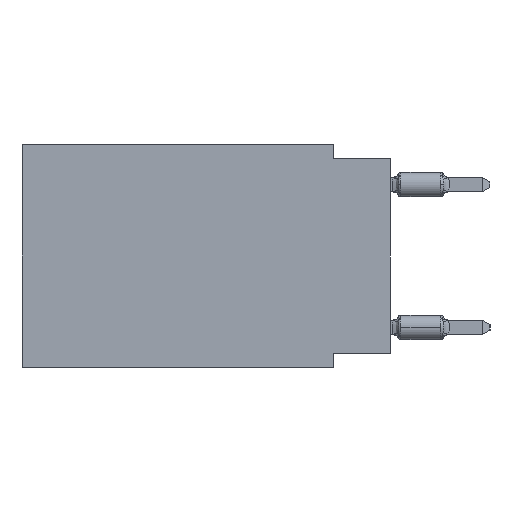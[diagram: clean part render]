
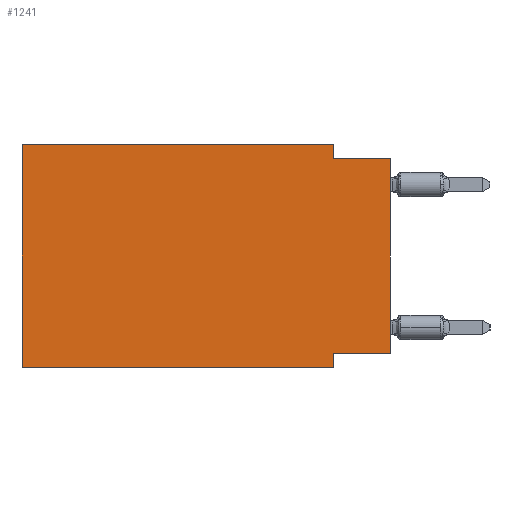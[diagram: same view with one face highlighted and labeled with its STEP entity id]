
A CAD part, left-side view. The second image highlights one B-rep face of the part: STEP entity #1241.
In plain terms, the highlighted planar face has unit normal (-1, 0, 0).
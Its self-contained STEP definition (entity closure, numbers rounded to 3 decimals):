
#1184 = DIRECTION ( 'NONE',  ( 0., 0., -1. ) ) ;
#1241 = ADVANCED_FACE ( 'NONE', ( #9945 ), #9842, .F. ) ;
#1271 = VERTEX_POINT ( 'NONE', #1636 ) ;
#1636 = CARTESIAN_POINT ( 'NONE',  ( 0., 16.383, -9.906 ) ) ;
#2718 = ORIENTED_EDGE ( 'NONE', *, *, #7008, .F. ) ;
#3216 = DIRECTION ( 'NONE',  ( 0., -1., 0. ) ) ;
#3234 = LINE ( 'NONE', #7346, #17052 ) ;
#3981 = ORIENTED_EDGE ( 'NONE', *, *, #22435, .F. ) ;
#5468 = CARTESIAN_POINT ( 'NONE',  ( 0., 2.54, -9.906 ) ) ;
#5648 = EDGE_CURVE ( 'NONE', #15885, #8867, #14203, .T. ) ;
#6075 = ORIENTED_EDGE ( 'NONE', *, *, #6110, .F. ) ;
#6110 = EDGE_CURVE ( 'NONE', #1271, #9626, #15998, .T. ) ;
#6120 = VERTEX_POINT ( 'NONE', #14290 ) ;
#6160 = VECTOR ( 'NONE', #12647, 1000. ) ;
#6846 = VECTOR ( 'NONE', #15282, 1000. ) ;
#6940 = DIRECTION ( 'NONE',  ( 0., -1., 0. ) ) ;
#7008 = EDGE_CURVE ( 'NONE', #9626, #15885, #8677, .T. ) ;
#7224 = DIRECTION ( 'NONE',  ( 0., 0., 1. ) ) ;
#7330 = EDGE_CURVE ( 'NONE', #7520, #19821, #3234, .T. ) ;
#7346 = CARTESIAN_POINT ( 'NONE',  ( 0., 0., 0. ) ) ;
#7520 = VERTEX_POINT ( 'NONE', #7574 ) ;
#7574 = CARTESIAN_POINT ( 'NONE',  ( 0., 0., -9.271 ) ) ;
#8401 = ORIENTED_EDGE ( 'NONE', *, *, #7330, .T. ) ;
#8583 = ORIENTED_EDGE ( 'NONE', *, *, #19744, .F. ) ;
#8677 = LINE ( 'NONE', #15727, #17412 ) ;
#8694 = VECTOR ( 'NONE', #3216, 1000. ) ;
#8867 = VERTEX_POINT ( 'NONE', #17205 ) ;
#8872 = DIRECTION ( 'NONE',  ( 0., 0., -1. ) ) ;
#8922 = VERTEX_POINT ( 'NONE', #15810 ) ;
#8942 = CARTESIAN_POINT ( 'NONE',  ( 0., 2.54, 0. ) ) ;
#9626 = VERTEX_POINT ( 'NONE', #10215 ) ;
#9842 = PLANE ( 'NONE',  #13290 ) ;
#9945 = FACE_OUTER_BOUND ( 'NONE', #11161, .T. ) ;
#10215 = CARTESIAN_POINT ( 'NONE',  ( 0., 16.383, 0. ) ) ;
#10247 = CARTESIAN_POINT ( 'NONE',  ( 0., 16.383, -9.906 ) ) ;
#10377 = EDGE_CURVE ( 'NONE', #1271, #6120, #13851, .T. ) ;
#10463 = CARTESIAN_POINT ( 'NONE',  ( 0., 16.383, 0. ) ) ;
#10715 = CARTESIAN_POINT ( 'NONE',  ( 0., 2.54, 0. ) ) ;
#11161 = EDGE_LOOP ( 'NONE', ( #8401, #8583, #22383, #2718, #6075, #17578, #22547, #3981 ) ) ;
#12647 = DIRECTION ( 'NONE',  ( 0., 0., -1. ) ) ;
#13290 = AXIS2_PLACEMENT_3D ( 'NONE', #16882, #16989, #1184 ) ;
#13450 = LINE ( 'NONE', #18965, #6846 ) ;
#13851 = LINE ( 'NONE', #10247, #8694 ) ;
#14203 = LINE ( 'NONE', #10715, #15516 ) ;
#14290 = CARTESIAN_POINT ( 'NONE',  ( 0., 2.54, -9.906 ) ) ;
#14982 = VECTOR ( 'NONE', #20389, 1000. ) ;
#15282 = DIRECTION ( 'NONE',  ( 0., -1., 0. ) ) ;
#15516 = VECTOR ( 'NONE', #8872, 1000. ) ;
#15592 = DIRECTION ( 'NONE',  ( 0., 0., 1. ) ) ;
#15727 = CARTESIAN_POINT ( 'NONE',  ( 0., 16.383, 0. ) ) ;
#15810 = CARTESIAN_POINT ( 'NONE',  ( 0., 2.54, -9.271 ) ) ;
#15885 = VERTEX_POINT ( 'NONE', #8942 ) ;
#15998 = LINE ( 'NONE', #10463, #16990 ) ;
#16586 = CARTESIAN_POINT ( 'NONE',  ( 0., 0., -9.271 ) ) ;
#16882 = CARTESIAN_POINT ( 'NONE',  ( 0., 16.383, 0. ) ) ;
#16989 = DIRECTION ( 'NONE',  ( 1., 0., 0. ) ) ;
#16990 = VECTOR ( 'NONE', #7224, 1000. ) ;
#17052 = VECTOR ( 'NONE', #15592, 1000. ) ;
#17205 = CARTESIAN_POINT ( 'NONE',  ( 0., 2.54, -0.635 ) ) ;
#17412 = VECTOR ( 'NONE', #6940, 1000. ) ;
#17578 = ORIENTED_EDGE ( 'NONE', *, *, #10377, .T. ) ;
#18150 = EDGE_CURVE ( 'NONE', #8922, #6120, #22748, .T. ) ;
#18629 = CARTESIAN_POINT ( 'NONE',  ( 0., 0., -0.635 ) ) ;
#18965 = CARTESIAN_POINT ( 'NONE',  ( 0., 0., -0.635 ) ) ;
#19744 = EDGE_CURVE ( 'NONE', #8867, #19821, #13450, .T. ) ;
#19821 = VERTEX_POINT ( 'NONE', #18629 ) ;
#19929 = LINE ( 'NONE', #16586, #14982 ) ;
#20389 = DIRECTION ( 'NONE',  ( 0., 1., 0. ) ) ;
#22383 = ORIENTED_EDGE ( 'NONE', *, *, #5648, .F. ) ;
#22435 = EDGE_CURVE ( 'NONE', #7520, #8922, #19929, .T. ) ;
#22547 = ORIENTED_EDGE ( 'NONE', *, *, #18150, .F. ) ;
#22748 = LINE ( 'NONE', #5468, #6160 ) ;
